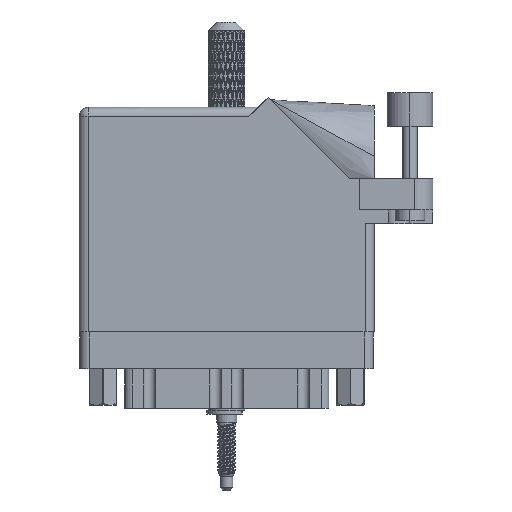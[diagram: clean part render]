
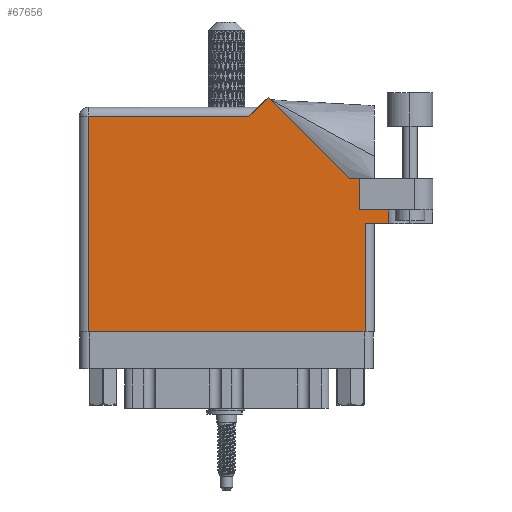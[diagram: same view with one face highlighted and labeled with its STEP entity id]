
A CAD part, front view. The second image highlights one B-rep face of the part: STEP entity #67656.
In plain terms, the highlighted face is planar.
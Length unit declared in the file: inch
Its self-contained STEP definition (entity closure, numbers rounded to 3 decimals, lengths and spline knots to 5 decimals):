
#764 = ORIENTED_EDGE ( 'NONE', *, *, #86832, .F. ) ;
#2005 = LINE ( 'NONE', #34251, #68178 ) ;
#3438 = VECTOR ( 'NONE', #18964, 39.37008 ) ;
#6355 = ORIENTED_EDGE ( 'NONE', *, *, #50210, .T. ) ;
#7207 = VECTOR ( 'NONE', #75499, 39.37008 ) ;
#7603 = EDGE_CURVE ( 'NONE', #81398, #96952, #18268, .T. ) ;
#9022 = VECTOR ( 'NONE', #24625, 39.37008 ) ;
#9810 = EDGE_CURVE ( 'NONE', #23525, #20043, #106433, .T. ) ;
#11535 = EDGE_CURVE ( 'NONE', #91061, #102297, #21918, .T. ) ;
#11727 = VERTEX_POINT ( 'NONE', #30384 ) ;
#12592 = CARTESIAN_POINT ( 'NONE',  ( 1.84442, 1.044, 0. ) ) ;
#14856 = PLANE ( 'NONE',  #103643 ) ;
#18268 = LINE ( 'NONE', #53246, #104727 ) ;
#18663 = VERTEX_POINT ( 'NONE', #103152 ) ;
#18731 = CARTESIAN_POINT ( 'NONE',  ( 1.84442, 1.044, 0. ) ) ;
#18964 = DIRECTION ( 'NONE',  ( -1., 0., 0. ) ) ;
#19147 = LINE ( 'NONE', #62458, #22740 ) ;
#20043 = VERTEX_POINT ( 'NONE', #12592 ) ;
#20329 = VERTEX_POINT ( 'NONE', #95229 ) ;
#21918 = LINE ( 'NONE', #30796, #59501 ) ;
#22600 = LINE ( 'NONE', #73093, #91806 ) ;
#22740 = VECTOR ( 'NONE', #70198, 39.37008 ) ;
#23525 = VERTEX_POINT ( 'NONE', #31425 ) ;
#24625 = DIRECTION ( 'NONE',  ( 1., 0., 0. ) ) ;
#27078 = LINE ( 'NONE', #18731, #43772 ) ;
#27808 = ORIENTED_EDGE ( 'NONE', *, *, #99211, .T. ) ;
#28595 = EDGE_CURVE ( 'NONE', #18663, #81398, #48538, .T. ) ;
#30384 = CARTESIAN_POINT ( 'NONE',  ( 0.062, 1.468, 0. ) ) ;
#30796 = CARTESIAN_POINT ( 'NONE',  ( 1.217, 1.53, 0. ) ) ;
#31326 = CARTESIAN_POINT ( 'NONE',  ( 0., 0., 0. ) ) ;
#31425 = CARTESIAN_POINT ( 'NONE',  ( 1.91, 1.044, 0. ) ) ;
#32662 = ORIENTED_EDGE ( 'NONE', *, *, #104674, .T. ) ;
#33316 = ORIENTED_EDGE ( 'NONE', *, *, #11535, .T. ) ;
#34251 = CARTESIAN_POINT ( 'NONE',  ( 1.91, 0.831, 0. ) ) ;
#36911 = DIRECTION ( 'NONE',  ( -0.707, -0.707, 0. ) ) ;
#38235 = EDGE_CURVE ( 'NONE', #106233, #20329, #19147, .T. ) ;
#40612 = VERTEX_POINT ( 'NONE', #76915 ) ;
#43660 = VECTOR ( 'NONE', #91953, 39.37008 ) ;
#43772 = VECTOR ( 'NONE', #44825, 39.37008 ) ;
#43957 = LINE ( 'NONE', #68388, #3438 ) ;
#44339 = DIRECTION ( 'NONE',  ( 1., 0., 0. ) ) ;
#44634 = ORIENTED_EDGE ( 'NONE', *, *, #46329, .T. ) ;
#44825 = DIRECTION ( 'NONE',  ( -0.707, 0.707, 0. ) ) ;
#46329 = EDGE_CURVE ( 'NONE', #11727, #18663, #22600, .T. ) ;
#48538 = LINE ( 'NONE', #31326, #9022 ) ;
#50210 = EDGE_CURVE ( 'NONE', #102297, #11727, #43957, .T. ) ;
#51482 = DIRECTION ( 'NONE',  ( 0., 1., 0. ) ) ;
#53246 = CARTESIAN_POINT ( 'NONE',  ( 1.948, 0.737, 0. ) ) ;
#55867 = CARTESIAN_POINT ( 'NONE',  ( 2.1115, 0.831, 0. ) ) ;
#59501 = VECTOR ( 'NONE', #36911, 39.37008 ) ;
#61122 = ORIENTED_EDGE ( 'NONE', *, *, #9810, .T. ) ;
#62458 = CARTESIAN_POINT ( 'NONE',  ( 2.1115, 1.16177, 0. ) ) ;
#64278 = FACE_OUTER_BOUND ( 'NONE', #81639, .T. ) ;
#65075 = CARTESIAN_POINT ( 'NONE',  ( 1.948, 0.737, 0. ) ) ;
#65869 = DIRECTION ( 'NONE',  ( 0., -1., 0. ) ) ;
#66108 = LINE ( 'NONE', #99999, #7207 ) ;
#67656 = ADVANCED_FACE ( 'NONE', ( #64278 ), #14856, .F. ) ;
#68178 = VECTOR ( 'NONE', #51482, 39.37008 ) ;
#68388 = CARTESIAN_POINT ( 'NONE',  ( 0., 1.468, 0. ) ) ;
#70198 = DIRECTION ( 'NONE',  ( 0., -1., 0. ) ) ;
#70380 = DIRECTION ( 'NONE',  ( 0., 1., 0. ) ) ;
#73093 = CARTESIAN_POINT ( 'NONE',  ( 0.062, 0., 0. ) ) ;
#73866 = EDGE_CURVE ( 'NONE', #96952, #20329, #66108, .T. ) ;
#74335 = CARTESIAN_POINT ( 'NONE',  ( 1.948, 0., 0. ) ) ;
#75499 = DIRECTION ( 'NONE',  ( 1., 0., 0. ) ) ;
#76395 = CARTESIAN_POINT ( 'NONE',  ( 1.155, 1.468, 0. ) ) ;
#76915 = CARTESIAN_POINT ( 'NONE',  ( 1.91, 0.831, 0. ) ) ;
#81398 = VERTEX_POINT ( 'NONE', #74335 ) ;
#81457 = CARTESIAN_POINT ( 'NONE',  ( 0., 1.53, 0. ) ) ;
#81639 = EDGE_LOOP ( 'NONE', ( #88939, #108502, #100187, #102921, #764, #27808, #61122, #32662, #33316, #6355, #44634 ) ) ;
#81997 = DIRECTION ( 'NONE',  ( 0., 0., -1. ) ) ;
#86832 = EDGE_CURVE ( 'NONE', #40612, #106233, #104827, .T. ) ;
#88939 = ORIENTED_EDGE ( 'NONE', *, *, #28595, .T. ) ;
#91061 = VERTEX_POINT ( 'NONE', #96755 ) ;
#91806 = VECTOR ( 'NONE', #65869, 39.37008 ) ;
#91953 = DIRECTION ( 'NONE',  ( -1., 0., 0. ) ) ;
#93066 = CARTESIAN_POINT ( 'NONE',  ( 2.41, 1.044, 0. ) ) ;
#95229 = CARTESIAN_POINT ( 'NONE',  ( 2.1115, 0.737, 0. ) ) ;
#96755 = CARTESIAN_POINT ( 'NONE',  ( 1.28771, 1.60071, 0. ) ) ;
#96952 = VERTEX_POINT ( 'NONE', #65075 ) ;
#99211 = EDGE_CURVE ( 'NONE', #40612, #23525, #2005, .T. ) ;
#99999 = CARTESIAN_POINT ( 'NONE',  ( 2.01, 0.737, 0. ) ) ;
#100187 = ORIENTED_EDGE ( 'NONE', *, *, #73866, .T. ) ;
#102297 = VERTEX_POINT ( 'NONE', #76395 ) ;
#102848 = VECTOR ( 'NONE', #44339, 39.37008 ) ;
#102921 = ORIENTED_EDGE ( 'NONE', *, *, #38235, .F. ) ;
#103152 = CARTESIAN_POINT ( 'NONE',  ( 0.062, 0., 0. ) ) ;
#103194 = CARTESIAN_POINT ( 'NONE',  ( 1.91, 0.831, 0. ) ) ;
#103643 = AXIS2_PLACEMENT_3D ( 'NONE', #81457, #81997, #106456 ) ;
#104674 = EDGE_CURVE ( 'NONE', #20043, #91061, #27078, .T. ) ;
#104727 = VECTOR ( 'NONE', #70380, 39.37008 ) ;
#104827 = LINE ( 'NONE', #103194, #102848 ) ;
#106233 = VERTEX_POINT ( 'NONE', #55867 ) ;
#106433 = LINE ( 'NONE', #93066, #43660 ) ;
#106456 = DIRECTION ( 'NONE',  ( -1., 0., 0. ) ) ;
#108502 = ORIENTED_EDGE ( 'NONE', *, *, #7603, .T. ) ;
